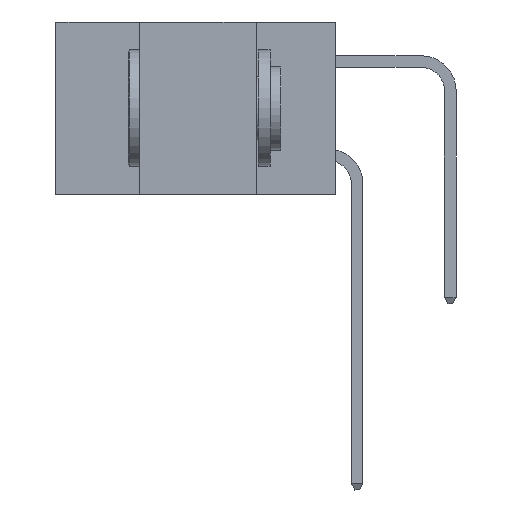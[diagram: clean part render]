
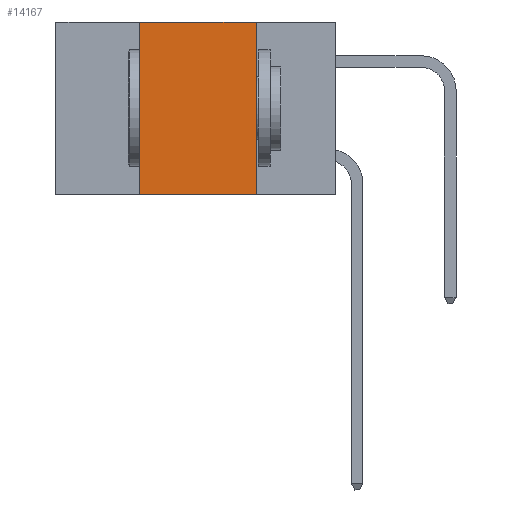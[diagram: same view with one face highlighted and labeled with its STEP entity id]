
A CAD part, left-side view. The second image highlights one B-rep face of the part: STEP entity #14167.
In plain terms, the highlighted planar face has unit normal (-1, 0, 0).
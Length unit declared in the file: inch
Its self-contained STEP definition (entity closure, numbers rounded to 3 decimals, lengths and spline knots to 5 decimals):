
#217 = VECTOR ( 'NONE', #3134, 39.37008 ) ;
#239 = VECTOR ( 'NONE', #19182, 39.37008 ) ;
#942 = EDGE_CURVE ( 'NONE', #10807, #11005, #15187, .T. ) ;
#1141 = VECTOR ( 'NONE', #3817, 39.37008 ) ;
#1145 = CARTESIAN_POINT ( 'NONE',  ( 0., 0.42, 0. ) ) ;
#1394 = EDGE_CURVE ( 'NONE', #11005, #15194, #10741, .T. ) ;
#2773 = VECTOR ( 'NONE', #23874, 39.37008 ) ;
#3134 = DIRECTION ( 'NONE',  ( 0., 0., -1. ) ) ;
#3448 = CARTESIAN_POINT ( 'NONE',  ( 0., 0.6, 0. ) ) ;
#3541 = PLANE ( 'NONE',  #18067 ) ;
#3817 = DIRECTION ( 'NONE',  ( 0., -1., 0. ) ) ;
#3958 = CARTESIAN_POINT ( 'NONE',  ( 0., 0.17, 0. ) ) ;
#5190 = CARTESIAN_POINT ( 'NONE',  ( 0., 0.17, -0.37 ) ) ;
#5582 = DIRECTION ( 'NONE',  ( 1., 0., 0. ) ) ;
#6506 = LINE ( 'NONE', #11670, #1141 ) ;
#7716 = EDGE_LOOP ( 'NONE', ( #9012, #21435, #15266, #15590 ) ) ;
#9012 = ORIENTED_EDGE ( 'NONE', *, *, #1394, .F. ) ;
#10741 = LINE ( 'NONE', #3958, #217 ) ;
#10807 = VERTEX_POINT ( 'NONE', #1145 ) ;
#11005 = VERTEX_POINT ( 'NONE', #20932 ) ;
#11278 = CARTESIAN_POINT ( 'NONE',  ( 0., 0.42, -0.37 ) ) ;
#11670 = CARTESIAN_POINT ( 'NONE',  ( 0., 0.6, -0.37 ) ) ;
#12664 = LINE ( 'NONE', #12699, #2773 ) ;
#12699 = CARTESIAN_POINT ( 'NONE',  ( 0., 0.42, 0. ) ) ;
#13245 = FACE_OUTER_BOUND ( 'NONE', #7716, .T. ) ;
#14167 = ADVANCED_FACE ( 'NONE', ( #13245 ), #3541, .F. ) ;
#15187 = LINE ( 'NONE', #19106, #239 ) ;
#15194 = VERTEX_POINT ( 'NONE', #5190 ) ;
#15266 = ORIENTED_EDGE ( 'NONE', *, *, #18755, .F. ) ;
#15590 = ORIENTED_EDGE ( 'NONE', *, *, #20914, .T. ) ;
#17090 = VERTEX_POINT ( 'NONE', #11278 ) ;
#18067 = AXIS2_PLACEMENT_3D ( 'NONE', #3448, #5582, #18967 ) ;
#18755 = EDGE_CURVE ( 'NONE', #17090, #10807, #12664, .T. ) ;
#18967 = DIRECTION ( 'NONE',  ( 0., 0., -1. ) ) ;
#19106 = CARTESIAN_POINT ( 'NONE',  ( 0., 0.6, 0. ) ) ;
#19182 = DIRECTION ( 'NONE',  ( 0., -1., 0. ) ) ;
#20914 = EDGE_CURVE ( 'NONE', #17090, #15194, #6506, .T. ) ;
#20932 = CARTESIAN_POINT ( 'NONE',  ( 0., 0.17, 0. ) ) ;
#21435 = ORIENTED_EDGE ( 'NONE', *, *, #942, .F. ) ;
#23874 = DIRECTION ( 'NONE',  ( 0., 0., 1. ) ) ;
